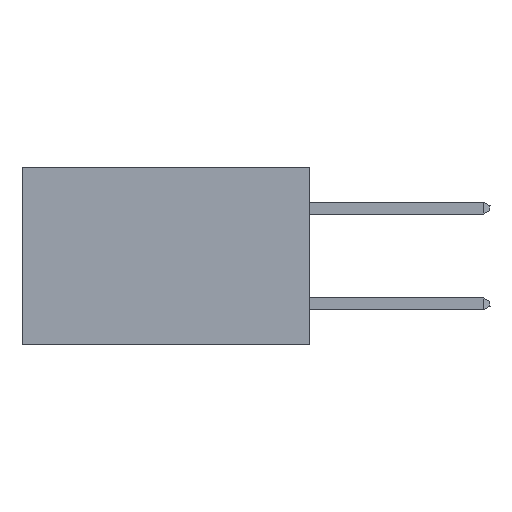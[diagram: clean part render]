
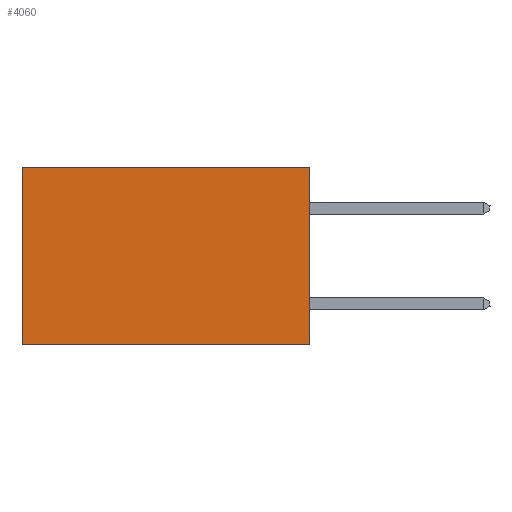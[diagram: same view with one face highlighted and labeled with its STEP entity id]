
A CAD part, left-side view. The second image highlights one B-rep face of the part: STEP entity #4060.
In plain terms, the highlighted planar face has unit normal (-1, 0, 0).
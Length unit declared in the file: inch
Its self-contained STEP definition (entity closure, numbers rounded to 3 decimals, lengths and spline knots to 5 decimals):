
#187 = CARTESIAN_POINT ( 'NONE',  ( 0.2875, 0.6, 0. ) ) ;
#339 = DIRECTION ( 'NONE',  ( 0., 0., -1. ) ) ;
#639 = CARTESIAN_POINT ( 'NONE',  ( 0.2875, 0.6, 0. ) ) ;
#816 = CARTESIAN_POINT ( 'NONE',  ( 0.2875, 0., 0. ) ) ;
#877 = EDGE_CURVE ( 'NONE', #2381, #4718, #5988, .T. ) ;
#1815 = EDGE_CURVE ( 'NONE', #15582, #12314, #6504, .T. ) ;
#2166 = ORIENTED_EDGE ( 'NONE', *, *, #2231, .T. ) ;
#2231 = EDGE_CURVE ( 'NONE', #12314, #4718, #5168, .T. ) ;
#2381 = VERTEX_POINT ( 'NONE', #11586 ) ;
#3407 = CARTESIAN_POINT ( 'NONE',  ( 0.2875, 0., -0.37 ) ) ;
#3645 = VECTOR ( 'NONE', #13827, 39.37008 ) ;
#3875 = VECTOR ( 'NONE', #10731, 39.37008 ) ;
#3970 = PLANE ( 'NONE',  #5344 ) ;
#4060 = ADVANCED_FACE ( 'NONE', ( #12558 ), #3970, .F. ) ;
#4718 = VERTEX_POINT ( 'NONE', #6327 ) ;
#5028 = ORIENTED_EDGE ( 'NONE', *, *, #8583, .F. ) ;
#5168 = LINE ( 'NONE', #639, #13217 ) ;
#5344 = AXIS2_PLACEMENT_3D ( 'NONE', #9946, #13785, #339 ) ;
#5976 = CARTESIAN_POINT ( 'NONE',  ( 0.2875, 0., 0. ) ) ;
#5988 = LINE ( 'NONE', #3407, #3875 ) ;
#6327 = CARTESIAN_POINT ( 'NONE',  ( 0.2875, 0.6, -0.37 ) ) ;
#6504 = LINE ( 'NONE', #13659, #3645 ) ;
#6653 = EDGE_LOOP ( 'NONE', ( #2166, #12146, #5028, #8415 ) ) ;
#7325 = LINE ( 'NONE', #5976, #12856 ) ;
#8415 = ORIENTED_EDGE ( 'NONE', *, *, #1815, .T. ) ;
#8583 = EDGE_CURVE ( 'NONE', #15582, #2381, #7325, .T. ) ;
#9946 = CARTESIAN_POINT ( 'NONE',  ( 0.2875, 0., 0. ) ) ;
#10400 = DIRECTION ( 'NONE',  ( 0., 0., -1. ) ) ;
#10731 = DIRECTION ( 'NONE',  ( 0., 1., 0. ) ) ;
#11586 = CARTESIAN_POINT ( 'NONE',  ( 0.2875, 0., -0.37 ) ) ;
#12146 = ORIENTED_EDGE ( 'NONE', *, *, #877, .F. ) ;
#12314 = VERTEX_POINT ( 'NONE', #187 ) ;
#12558 = FACE_OUTER_BOUND ( 'NONE', #6653, .T. ) ;
#12856 = VECTOR ( 'NONE', #15667, 39.37008 ) ;
#13217 = VECTOR ( 'NONE', #10400, 39.37008 ) ;
#13659 = CARTESIAN_POINT ( 'NONE',  ( 0.2875, 0., 0. ) ) ;
#13785 = DIRECTION ( 'NONE',  ( 1., 0., 0. ) ) ;
#13827 = DIRECTION ( 'NONE',  ( 0., 1., 0. ) ) ;
#15582 = VERTEX_POINT ( 'NONE', #816 ) ;
#15667 = DIRECTION ( 'NONE',  ( 0., 0., -1. ) ) ;
